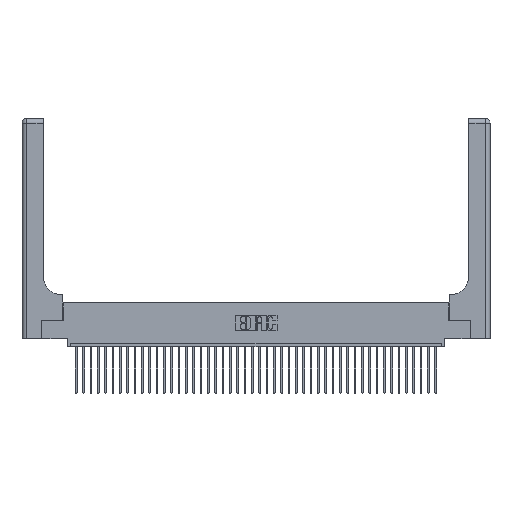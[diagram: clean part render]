
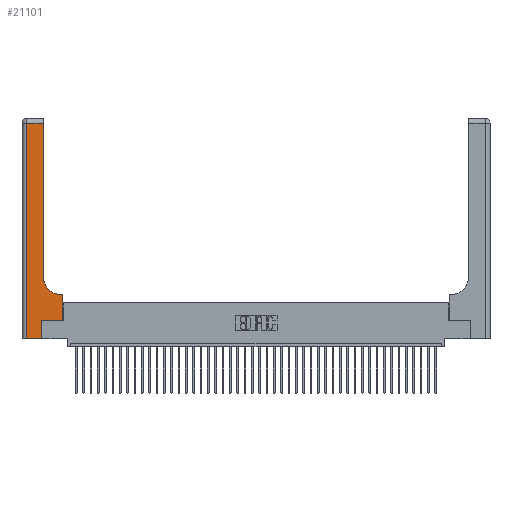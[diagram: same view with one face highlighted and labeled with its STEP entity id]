
A CAD part, top view. The second image highlights one B-rep face of the part: STEP entity #21101.
In plain terms, the highlighted planar face has unit normal (0, 0, 1).
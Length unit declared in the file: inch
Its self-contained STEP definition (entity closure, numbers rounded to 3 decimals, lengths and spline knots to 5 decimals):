
#644 = CIRCLE ( 'NONE', #40736, 0.25 ) ;
#1049 = LINE ( 'NONE', #16628, #3143 ) ;
#1999 = AXIS2_PLACEMENT_3D ( 'NONE', #29106, #39241, #23121 ) ;
#2071 = EDGE_CURVE ( 'NONE', #19835, #16990, #2633, .T. ) ;
#2633 = LINE ( 'NONE', #4110, #36957 ) ;
#2944 = DIRECTION ( 'NONE',  ( -1., 0., 0. ) ) ;
#3143 = VECTOR ( 'NONE', #13534, 39.37008 ) ;
#3696 = EDGE_LOOP ( 'NONE', ( #18985, #11969, #14272, #29896, #12595, #35633, #16930, #22147, #6075 ) ) ;
#3868 = CARTESIAN_POINT ( 'NONE',  ( 0.06, 3., 0.37 ) ) ;
#4110 = CARTESIAN_POINT ( 'NONE',  ( 0.2915, 3., 0.37 ) ) ;
#5444 = DIRECTION ( 'NONE',  ( 1., 0., 0. ) ) ;
#5606 = EDGE_CURVE ( 'NONE', #40224, #9917, #35430, .T. ) ;
#5761 = LINE ( 'NONE', #28501, #27435 ) ;
#6075 = ORIENTED_EDGE ( 'NONE', *, *, #14321, .T. ) ;
#6219 = CARTESIAN_POINT ( 'NONE',  ( 0.269, 0., 0.37 ) ) ;
#7229 = DIRECTION ( 'NONE',  ( 0., 1., 0. ) ) ;
#7436 = DIRECTION ( 'NONE',  ( 0., -1., 0. ) ) ;
#7542 = CARTESIAN_POINT ( 'NONE',  ( 0.06, 2.94, 0.37 ) ) ;
#7682 = EDGE_CURVE ( 'NONE', #28646, #29847, #13532, .T. ) ;
#8221 = CARTESIAN_POINT ( 'NONE',  ( 0., 0., 0.37 ) ) ;
#9917 = VERTEX_POINT ( 'NONE', #33077 ) ;
#10802 = EDGE_CURVE ( 'NONE', #17949, #40224, #26948, .T. ) ;
#11969 = ORIENTED_EDGE ( 'NONE', *, *, #34901, .T. ) ;
#12379 = DIRECTION ( 'NONE',  ( 0., 0., -1. ) ) ;
#12595 = ORIENTED_EDGE ( 'NONE', *, *, #34915, .T. ) ;
#12632 = CARTESIAN_POINT ( 'NONE',  ( 0.5585, 0.6, 0.37 ) ) ;
#13532 = LINE ( 'NONE', #33990, #14582 ) ;
#13534 = DIRECTION ( 'NONE',  ( -1., 0., 0. ) ) ;
#14272 = ORIENTED_EDGE ( 'NONE', *, *, #10802, .T. ) ;
#14321 = EDGE_CURVE ( 'NONE', #36466, #19835, #644, .T. ) ;
#14582 = VECTOR ( 'NONE', #34137, 39.37008 ) ;
#15405 = CARTESIAN_POINT ( 'NONE',  ( 0.5585, 0.25, 0.37 ) ) ;
#15779 = VECTOR ( 'NONE', #30798, 39.37008 ) ;
#16628 = CARTESIAN_POINT ( 'NONE',  ( 0.2915, 0.6, 0.37 ) ) ;
#16930 = ORIENTED_EDGE ( 'NONE', *, *, #7682, .T. ) ;
#16990 = VERTEX_POINT ( 'NONE', #34529 ) ;
#17000 = VECTOR ( 'NONE', #25012, 39.37008 ) ;
#17949 = VERTEX_POINT ( 'NONE', #7542 ) ;
#18448 = VERTEX_POINT ( 'NONE', #33958 ) ;
#18867 = CARTESIAN_POINT ( 'NONE',  ( 0.5415, 0.85, 0.37 ) ) ;
#18985 = ORIENTED_EDGE ( 'NONE', *, *, #2071, .T. ) ;
#19835 = VERTEX_POINT ( 'NONE', #36444 ) ;
#20855 = CARTESIAN_POINT ( 'NONE',  ( 0.269, 0.25, 0.37 ) ) ;
#21101 = ADVANCED_FACE ( 'NONE', ( #26459 ), #29236, .F. ) ;
#22147 = ORIENTED_EDGE ( 'NONE', *, *, #41677, .T. ) ;
#22412 = LINE ( 'NONE', #6219, #39036 ) ;
#23121 = DIRECTION ( 'NONE',  ( -1., 0., 0. ) ) ;
#25012 = DIRECTION ( 'NONE',  ( 1., 0., 0. ) ) ;
#26076 = LINE ( 'NONE', #20855, #17000 ) ;
#26459 = FACE_OUTER_BOUND ( 'NONE', #3696, .T. ) ;
#26948 = LINE ( 'NONE', #3868, #34037 ) ;
#27435 = VECTOR ( 'NONE', #2944, 39.37008 ) ;
#27496 = CARTESIAN_POINT ( 'NONE',  ( 0.5415, 0.6, 0.37 ) ) ;
#28501 = CARTESIAN_POINT ( 'NONE',  ( 0., 2.94, 0.37 ) ) ;
#28646 = VERTEX_POINT ( 'NONE', #15405 ) ;
#29106 = CARTESIAN_POINT ( 'NONE',  ( 0., 3., 0.37 ) ) ;
#29236 = PLANE ( 'NONE',  #1999 ) ;
#29847 = VERTEX_POINT ( 'NONE', #12632 ) ;
#29896 = ORIENTED_EDGE ( 'NONE', *, *, #5606, .T. ) ;
#30798 = DIRECTION ( 'NONE',  ( 1., 0., 0. ) ) ;
#33077 = CARTESIAN_POINT ( 'NONE',  ( 0.269, 0., 0.37 ) ) ;
#33958 = CARTESIAN_POINT ( 'NONE',  ( 0.269, 0.25, 0.37 ) ) ;
#33990 = CARTESIAN_POINT ( 'NONE',  ( 0.5585, 0.25, 0.37 ) ) ;
#34037 = VECTOR ( 'NONE', #7436, 39.37008 ) ;
#34137 = DIRECTION ( 'NONE',  ( 0., 1., 0. ) ) ;
#34529 = CARTESIAN_POINT ( 'NONE',  ( 0.2915, 2.94, 0.37 ) ) ;
#34901 = EDGE_CURVE ( 'NONE', #16990, #17949, #5761, .T. ) ;
#34915 = EDGE_CURVE ( 'NONE', #9917, #18448, #22412, .T. ) ;
#35430 = LINE ( 'NONE', #8221, #15779 ) ;
#35633 = ORIENTED_EDGE ( 'NONE', *, *, #38945, .T. ) ;
#36444 = CARTESIAN_POINT ( 'NONE',  ( 0.2915, 0.85, 0.37 ) ) ;
#36466 = VERTEX_POINT ( 'NONE', #27496 ) ;
#36957 = VECTOR ( 'NONE', #7229, 39.37008 ) ;
#38945 = EDGE_CURVE ( 'NONE', #18448, #28646, #26076, .T. ) ;
#39036 = VECTOR ( 'NONE', #41551, 39.37008 ) ;
#39241 = DIRECTION ( 'NONE',  ( 0., 0., -1. ) ) ;
#40224 = VERTEX_POINT ( 'NONE', #40987 ) ;
#40736 = AXIS2_PLACEMENT_3D ( 'NONE', #18867, #12379, #5444 ) ;
#40987 = CARTESIAN_POINT ( 'NONE',  ( 0.06, 0., 0.37 ) ) ;
#41551 = DIRECTION ( 'NONE',  ( 0., 1., 0. ) ) ;
#41677 = EDGE_CURVE ( 'NONE', #29847, #36466, #1049, .T. ) ;
